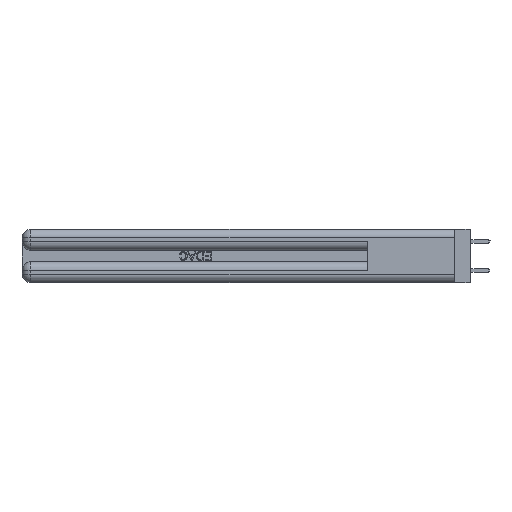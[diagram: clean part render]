
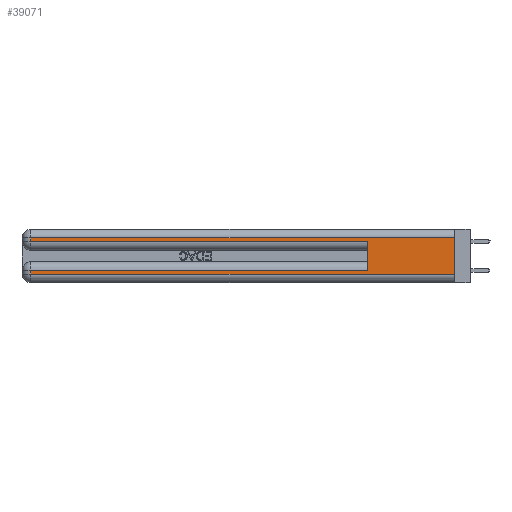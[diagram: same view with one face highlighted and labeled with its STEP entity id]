
A CAD part, left-side view. The second image highlights one B-rep face of the part: STEP entity #39071.
In plain terms, the highlighted planar face has unit normal (-1, 0, 0).
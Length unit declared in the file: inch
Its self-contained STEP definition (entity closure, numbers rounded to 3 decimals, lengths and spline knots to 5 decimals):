
#378 = ORIENTED_EDGE ( 'NONE', *, *, #27438, .T. ) ;
#639 = LINE ( 'NONE', #26299, #38453 ) ;
#2179 = CARTESIAN_POINT ( 'NONE',  ( 0., 2.94, 0.31 ) ) ;
#2810 = DIRECTION ( 'NONE',  ( 0., 0., 1. ) ) ;
#3087 = PLANE ( 'NONE',  #36988 ) ;
#3958 = ORIENTED_EDGE ( 'NONE', *, *, #16690, .T. ) ;
#4124 = LINE ( 'NONE', #43806, #41883 ) ;
#8016 = CARTESIAN_POINT ( 'NONE',  ( 0., 0., 0.06 ) ) ;
#8207 = ORIENTED_EDGE ( 'NONE', *, *, #30588, .T. ) ;
#9418 = CARTESIAN_POINT ( 'NONE',  ( 0., 0., 0.31 ) ) ;
#10191 = VECTOR ( 'NONE', #15075, 39.37008 ) ;
#10636 = EDGE_CURVE ( 'NONE', #42697, #26032, #13091, .T. ) ;
#12714 = LINE ( 'NONE', #26628, #30996 ) ;
#13091 = LINE ( 'NONE', #35913, #14260 ) ;
#13988 = VECTOR ( 'NONE', #21007, 39.37008 ) ;
#14260 = VECTOR ( 'NONE', #25121, 39.37008 ) ;
#14269 = DIRECTION ( 'NONE',  ( 1., 0., 0. ) ) ;
#14575 = CARTESIAN_POINT ( 'NONE',  ( 0., 2.94, 0.085 ) ) ;
#14759 = VECTOR ( 'NONE', #2810, 39.37008 ) ;
#15075 = DIRECTION ( 'NONE',  ( 0., -1., 0. ) ) ;
#16690 = EDGE_CURVE ( 'NONE', #46162, #27753, #639, .T. ) ;
#18705 = ORIENTED_EDGE ( 'NONE', *, *, #10636, .T. ) ;
#20527 = DIRECTION ( 'NONE',  ( 0., 1., 0. ) ) ;
#21007 = DIRECTION ( 'NONE',  ( 0., 0., -1. ) ) ;
#22197 = CARTESIAN_POINT ( 'NONE',  ( 0., 0.6, 0.085 ) ) ;
#23007 = CARTESIAN_POINT ( 'NONE',  ( 0., 2.94, 0.06 ) ) ;
#23762 = LINE ( 'NONE', #9418, #31140 ) ;
#24452 = LINE ( 'NONE', #43000, #14759 ) ;
#24730 = ORIENTED_EDGE ( 'NONE', *, *, #40659, .F. ) ;
#25121 = DIRECTION ( 'NONE',  ( 0., -1., 0. ) ) ;
#26032 = VERTEX_POINT ( 'NONE', #27006 ) ;
#26197 = CARTESIAN_POINT ( 'NONE',  ( 0., 0., 0.31 ) ) ;
#26299 = CARTESIAN_POINT ( 'NONE',  ( 0., 0., 0.085 ) ) ;
#26628 = CARTESIAN_POINT ( 'NONE',  ( 0., 2.94, 0.37 ) ) ;
#27006 = CARTESIAN_POINT ( 'NONE',  ( 0., 0.6, 0.285 ) ) ;
#27438 = EDGE_CURVE ( 'NONE', #32610, #32847, #23762, .T. ) ;
#27753 = VERTEX_POINT ( 'NONE', #14575 ) ;
#28311 = CARTESIAN_POINT ( 'NONE',  ( 0., 0., 0.37 ) ) ;
#29333 = DIRECTION ( 'NONE',  ( 0., 0., -1. ) ) ;
#29408 = ORIENTED_EDGE ( 'NONE', *, *, #35865, .F. ) ;
#29650 = LINE ( 'NONE', #40546, #10191 ) ;
#29972 = DIRECTION ( 'NONE',  ( 0., 1., 0. ) ) ;
#30588 = EDGE_CURVE ( 'NONE', #32847, #42697, #12714, .T. ) ;
#30782 = FACE_OUTER_BOUND ( 'NONE', #42293, .T. ) ;
#30996 = VECTOR ( 'NONE', #44920, 39.37008 ) ;
#31140 = VECTOR ( 'NONE', #20527, 39.37008 ) ;
#32241 = LINE ( 'NONE', #28311, #13988 ) ;
#32610 = VERTEX_POINT ( 'NONE', #26197 ) ;
#32847 = VERTEX_POINT ( 'NONE', #2179 ) ;
#35865 = EDGE_CURVE ( 'NONE', #32610, #46271, #32241, .T. ) ;
#35913 = CARTESIAN_POINT ( 'NONE',  ( 0., 0., 0.285 ) ) ;
#36096 = CARTESIAN_POINT ( 'NONE',  ( 0., 0., 0.37 ) ) ;
#36988 = AXIS2_PLACEMENT_3D ( 'NONE', #36096, #14269, #39760 ) ;
#38453 = VECTOR ( 'NONE', #29972, 39.37008 ) ;
#39071 = ADVANCED_FACE ( 'NONE', ( #30782 ), #3087, .F. ) ;
#39385 = ORIENTED_EDGE ( 'NONE', *, *, #41566, .T. ) ;
#39760 = DIRECTION ( 'NONE',  ( 0., 0., -1. ) ) ;
#40546 = CARTESIAN_POINT ( 'NONE',  ( 0., 0., 0.06 ) ) ;
#40659 = EDGE_CURVE ( 'NONE', #46162, #26032, #24452, .T. ) ;
#41566 = EDGE_CURVE ( 'NONE', #42320, #46271, #29650, .T. ) ;
#41883 = VECTOR ( 'NONE', #29333, 39.37008 ) ;
#42293 = EDGE_LOOP ( 'NONE', ( #29408, #378, #8207, #18705, #24730, #3958, #43533, #39385 ) ) ;
#42320 = VERTEX_POINT ( 'NONE', #23007 ) ;
#42697 = VERTEX_POINT ( 'NONE', #43629 ) ;
#43000 = CARTESIAN_POINT ( 'NONE',  ( 0., 0.6, 0.145 ) ) ;
#43533 = ORIENTED_EDGE ( 'NONE', *, *, #45131, .T. ) ;
#43629 = CARTESIAN_POINT ( 'NONE',  ( 0., 2.94, 0.285 ) ) ;
#43806 = CARTESIAN_POINT ( 'NONE',  ( 0., 2.94, 0.37 ) ) ;
#44920 = DIRECTION ( 'NONE',  ( 0., 0., -1. ) ) ;
#45131 = EDGE_CURVE ( 'NONE', #27753, #42320, #4124, .T. ) ;
#46162 = VERTEX_POINT ( 'NONE', #22197 ) ;
#46271 = VERTEX_POINT ( 'NONE', #8016 ) ;
